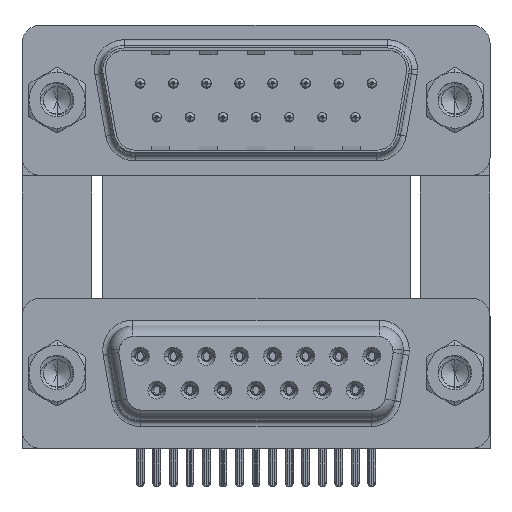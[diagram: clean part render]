
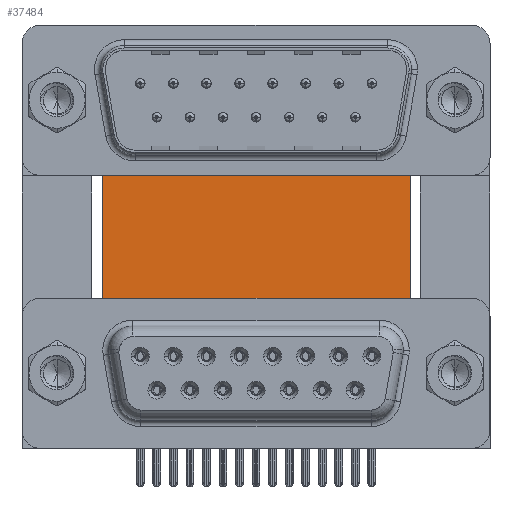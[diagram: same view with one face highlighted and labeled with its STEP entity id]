
A CAD part, top view. The second image highlights one B-rep face of the part: STEP entity #37484.
In plain terms, the highlighted planar face has unit normal (0, 0, 1).
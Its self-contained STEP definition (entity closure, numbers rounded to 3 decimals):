
#1665 = VECTOR ( 'NONE', #33444, 1000. ) ;
#2177 = DIRECTION ( 'NONE',  ( -1., 0., 0. ) ) ;
#2409 = LINE ( 'NONE', #32063, #4188 ) ;
#3052 = LINE ( 'NONE', #21326, #1665 ) ;
#4188 = VECTOR ( 'NONE', #47620, 1000. ) ;
#4230 = LINE ( 'NONE', #4476, #14042 ) ;
#4476 = CARTESIAN_POINT ( 'NONE',  ( 3.79, 16.585, -12. ) ) ;
#4865 = LINE ( 'NONE', #31280, #11943 ) ;
#6290 = EDGE_LOOP ( 'NONE', ( #11230, #25645, #26377, #44056 ) ) ;
#8045 = CARTESIAN_POINT ( 'NONE',  ( 29.58, 16.585, -12. ) ) ;
#8067 = DIRECTION ( 'NONE',  ( 1., 0., 0. ) ) ;
#8075 = EDGE_CURVE ( 'NONE', #21472, #31915, #3052, .T. ) ;
#11230 = ORIENTED_EDGE ( 'NONE', *, *, #8075, .T. ) ;
#11943 = VECTOR ( 'NONE', #8067, 1000. ) ;
#14042 = VECTOR ( 'NONE', #18773, 1000. ) ;
#16722 = DIRECTION ( 'NONE',  ( 0., 0., -1. ) ) ;
#18773 = DIRECTION ( 'NONE',  ( 0., -1., 0. ) ) ;
#21326 = CARTESIAN_POINT ( 'NONE',  ( 3.79, -3.735, -12. ) ) ;
#21472 = VERTEX_POINT ( 'NONE', #33568 ) ;
#25645 = ORIENTED_EDGE ( 'NONE', *, *, #42650, .F. ) ;
#26377 = ORIENTED_EDGE ( 'NONE', *, *, #28025, .F. ) ;
#27845 = FACE_OUTER_BOUND ( 'NONE', #6290, .T. ) ;
#28025 = EDGE_CURVE ( 'NONE', #40018, #42768, #4865, .T. ) ;
#28432 = AXIS2_PLACEMENT_3D ( 'NONE', #35522, #16722, #2177 ) ;
#31280 = CARTESIAN_POINT ( 'NONE',  ( 3.79, 16.585, -12. ) ) ;
#31915 = VERTEX_POINT ( 'NONE', #42367 ) ;
#32063 = CARTESIAN_POINT ( 'NONE',  ( 29.58, 16.585, -12. ) ) ;
#33444 = DIRECTION ( 'NONE',  ( 1., 0., 0. ) ) ;
#33568 = CARTESIAN_POINT ( 'NONE',  ( 3.79, -3.735, -12. ) ) ;
#33716 = EDGE_CURVE ( 'NONE', #40018, #21472, #4230, .T. ) ;
#35522 = CARTESIAN_POINT ( 'NONE',  ( 3.79, 16.585, -12. ) ) ;
#37484 = ADVANCED_FACE ( 'NONE', ( #27845 ), #43672, .F. ) ;
#40018 = VERTEX_POINT ( 'NONE', #41797 ) ;
#41797 = CARTESIAN_POINT ( 'NONE',  ( 3.79, 16.585, -12. ) ) ;
#42367 = CARTESIAN_POINT ( 'NONE',  ( 29.58, -3.735, -12. ) ) ;
#42650 = EDGE_CURVE ( 'NONE', #42768, #31915, #2409, .T. ) ;
#42768 = VERTEX_POINT ( 'NONE', #8045 ) ;
#43672 = PLANE ( 'NONE',  #28432 ) ;
#44056 = ORIENTED_EDGE ( 'NONE', *, *, #33716, .T. ) ;
#47620 = DIRECTION ( 'NONE',  ( 0., -1., 0. ) ) ;
